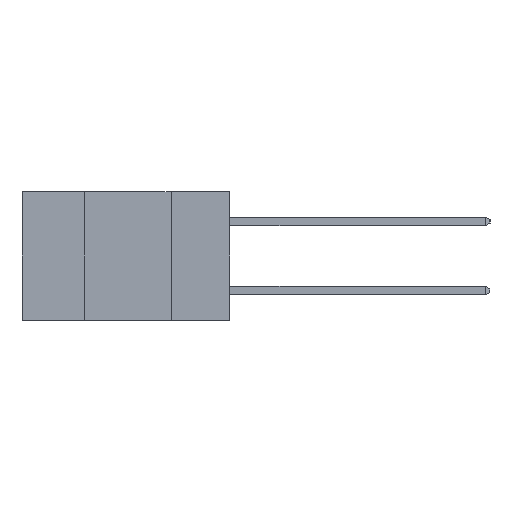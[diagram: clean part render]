
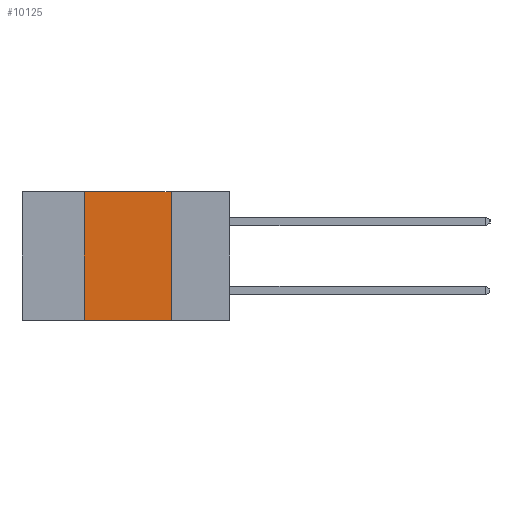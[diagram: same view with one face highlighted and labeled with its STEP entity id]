
A CAD part, left-side view. The second image highlights one B-rep face of the part: STEP entity #10125.
In plain terms, the highlighted planar face has unit normal (-1, 0, 0).
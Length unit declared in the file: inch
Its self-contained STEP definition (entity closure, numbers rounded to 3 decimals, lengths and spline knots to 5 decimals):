
#586 = CARTESIAN_POINT ( 'NONE',  ( 0., 0.42, 0. ) ) ;
#1019 = DIRECTION ( 'NONE',  ( 0., 0., -1. ) ) ;
#1137 = VERTEX_POINT ( 'NONE', #5482 ) ;
#1800 = VECTOR ( 'NONE', #1019, 39.37008 ) ;
#1969 = CARTESIAN_POINT ( 'NONE',  ( 0., 0.6, 0. ) ) ;
#2721 = FACE_OUTER_BOUND ( 'NONE', #3217, .T. ) ;
#2795 = CARTESIAN_POINT ( 'NONE',  ( 0., 0.42, -0.37 ) ) ;
#2969 = DIRECTION ( 'NONE',  ( 0., 0., -1. ) ) ;
#3217 = EDGE_LOOP ( 'NONE', ( #8332, #3481, #11360, #9776 ) ) ;
#3481 = ORIENTED_EDGE ( 'NONE', *, *, #8633, .F. ) ;
#3678 = AXIS2_PLACEMENT_3D ( 'NONE', #1969, #8764, #2969 ) ;
#3850 = VECTOR ( 'NONE', #7485, 39.37008 ) ;
#4130 = LINE ( 'NONE', #6056, #1800 ) ;
#4181 = LINE ( 'NONE', #10208, #9831 ) ;
#4405 = CARTESIAN_POINT ( 'NONE',  ( 0., 0.6, 0. ) ) ;
#5181 = CARTESIAN_POINT ( 'NONE',  ( 0., 0.17, 0. ) ) ;
#5482 = CARTESIAN_POINT ( 'NONE',  ( 0., 0.42, 0. ) ) ;
#5530 = DIRECTION ( 'NONE',  ( 0., -1., 0. ) ) ;
#5549 = EDGE_CURVE ( 'NONE', #8246, #6180, #4181, .T. ) ;
#5564 = EDGE_CURVE ( 'NONE', #8246, #1137, #7101, .T. ) ;
#6056 = CARTESIAN_POINT ( 'NONE',  ( 0., 0.17, 0. ) ) ;
#6180 = VERTEX_POINT ( 'NONE', #7391 ) ;
#6911 = PLANE ( 'NONE',  #3678 ) ;
#7101 = LINE ( 'NONE', #586, #3850 ) ;
#7353 = DIRECTION ( 'NONE',  ( 0., -1., 0. ) ) ;
#7391 = CARTESIAN_POINT ( 'NONE',  ( 0., 0.17, -0.37 ) ) ;
#7485 = DIRECTION ( 'NONE',  ( 0., 0., 1. ) ) ;
#8246 = VERTEX_POINT ( 'NONE', #2795 ) ;
#8332 = ORIENTED_EDGE ( 'NONE', *, *, #10220, .F. ) ;
#8633 = EDGE_CURVE ( 'NONE', #1137, #12151, #9172, .T. ) ;
#8764 = DIRECTION ( 'NONE',  ( 1., 0., 0. ) ) ;
#9172 = LINE ( 'NONE', #4405, #11045 ) ;
#9776 = ORIENTED_EDGE ( 'NONE', *, *, #5549, .T. ) ;
#9831 = VECTOR ( 'NONE', #5530, 39.37008 ) ;
#10125 = ADVANCED_FACE ( 'NONE', ( #2721 ), #6911, .F. ) ;
#10208 = CARTESIAN_POINT ( 'NONE',  ( 0., 0.6, -0.37 ) ) ;
#10220 = EDGE_CURVE ( 'NONE', #12151, #6180, #4130, .T. ) ;
#11045 = VECTOR ( 'NONE', #7353, 39.37008 ) ;
#11360 = ORIENTED_EDGE ( 'NONE', *, *, #5564, .F. ) ;
#12151 = VERTEX_POINT ( 'NONE', #5181 ) ;
